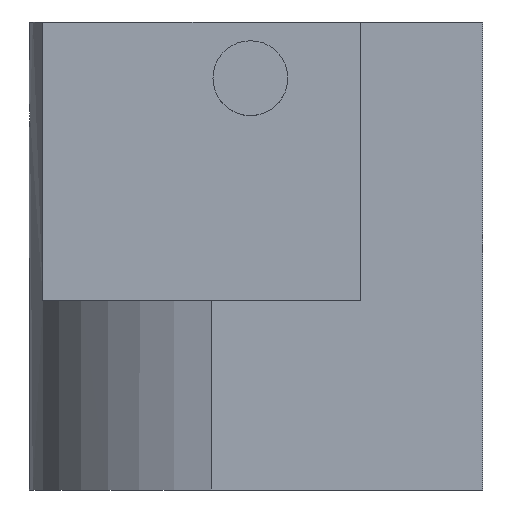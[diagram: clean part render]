
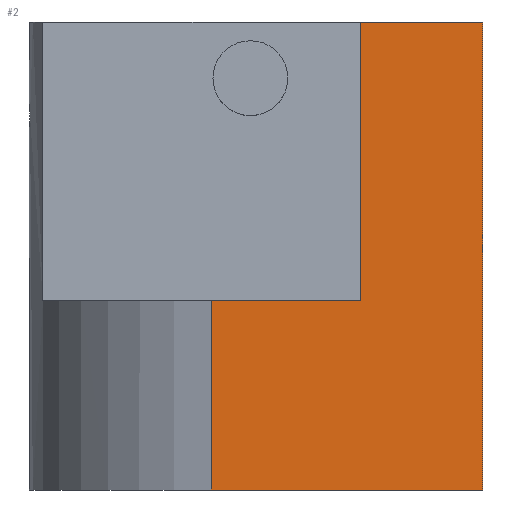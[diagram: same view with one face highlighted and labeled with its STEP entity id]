
A CAD part, left-side view. The second image highlights one B-rep face of the part: STEP entity #2.
In plain terms, the highlighted planar face has unit normal (-1, 0, 0).
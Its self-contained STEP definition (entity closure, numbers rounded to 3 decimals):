
#2 = ADVANCED_FACE ( 'NONE', ( #112 ), #1020, .F. ) ;
#26 = ORIENTED_EDGE ( 'NONE', *, *, #1511, .F. ) ;
#98 = VERTEX_POINT ( 'NONE', #1521 ) ;
#99 = LINE ( 'NONE', #606, #130 ) ;
#102 = DIRECTION ( 'NONE',  ( 0., 0., 1. ) ) ;
#106 = EDGE_LOOP ( 'NONE', ( #1433, #1058, #26, #1536, #1335, #1296 ) ) ;
#112 = FACE_OUTER_BOUND ( 'NONE', #106, .T. ) ;
#130 = VECTOR ( 'NONE', #1108, 1000. ) ;
#151 = CARTESIAN_POINT ( 'NONE',  ( -58.909, 11.39, -190. ) ) ;
#162 = CARTESIAN_POINT ( 'NONE',  ( -58.909, 11.39, -190. ) ) ;
#211 = DIRECTION ( 'NONE',  ( 0., 1., 0. ) ) ;
#288 = CARTESIAN_POINT ( 'NONE',  ( -58.909, -61., -65. ) ) ;
#294 = LINE ( 'NONE', #162, #819 ) ;
#301 = LINE ( 'NONE', #151, #1071 ) ;
#314 = VECTOR ( 'NONE', #211, 1000. ) ;
#342 = VERTEX_POINT ( 'NONE', #598 ) ;
#349 = CARTESIAN_POINT ( 'NONE',  ( -58.909, -28.313, -40. ) ) ;
#363 = AXIS2_PLACEMENT_3D ( 'NONE', #1121, #1144, #387 ) ;
#370 = EDGE_CURVE ( 'NONE', #1182, #448, #1351, .T. ) ;
#387 = DIRECTION ( 'NONE',  ( 0., 1., 0. ) ) ;
#395 = DIRECTION ( 'NONE',  ( 0., -1., 0. ) ) ;
#397 = VERTEX_POINT ( 'NONE', #1469 ) ;
#448 = VERTEX_POINT ( 'NONE', #887 ) ;
#529 = EDGE_CURVE ( 'NONE', #342, #1325, #294, .T. ) ;
#552 = DIRECTION ( 'NONE',  ( 0., 1., 0. ) ) ;
#598 = CARTESIAN_POINT ( 'NONE',  ( -58.909, -61., -190. ) ) ;
#606 = CARTESIAN_POINT ( 'NONE',  ( -58.909, -61., -190. ) ) ;
#780 = EDGE_CURVE ( 'NONE', #342, #1182, #99, .T. ) ;
#819 = VECTOR ( 'NONE', #552, 1000. ) ;
#821 = VECTOR ( 'NONE', #395, 1000. ) ;
#834 = CARTESIAN_POINT ( 'NONE',  ( -58.909, 11.39, -65. ) ) ;
#887 = CARTESIAN_POINT ( 'NONE',  ( -58.909, -28.313, -65. ) ) ;
#1019 = CARTESIAN_POINT ( 'NONE',  ( -58.909, -28.313, -139.424 ) ) ;
#1020 = PLANE ( 'NONE',  #363 ) ;
#1058 = ORIENTED_EDGE ( 'NONE', *, *, #1318, .F. ) ;
#1071 = VECTOR ( 'NONE', #1309, 1000. ) ;
#1108 = DIRECTION ( 'NONE',  ( 0., 0., 1. ) ) ;
#1121 = CARTESIAN_POINT ( 'NONE',  ( -58.909, 11.39, -190. ) ) ;
#1135 = LINE ( 'NONE', #1019, #821 ) ;
#1144 = DIRECTION ( 'NONE',  ( 1., 0., 0. ) ) ;
#1182 = VERTEX_POINT ( 'NONE', #288 ) ;
#1199 = CARTESIAN_POINT ( 'NONE',  ( -58.909, 11.39, -190. ) ) ;
#1296 = ORIENTED_EDGE ( 'NONE', *, *, #780, .T. ) ;
#1309 = DIRECTION ( 'NONE',  ( 0., 0., 1. ) ) ;
#1318 = EDGE_CURVE ( 'NONE', #397, #448, #1455, .T. ) ;
#1325 = VERTEX_POINT ( 'NONE', #1199 ) ;
#1335 = ORIENTED_EDGE ( 'NONE', *, *, #529, .F. ) ;
#1351 = LINE ( 'NONE', #834, #314 ) ;
#1433 = ORIENTED_EDGE ( 'NONE', *, *, #370, .T. ) ;
#1455 = LINE ( 'NONE', #349, #1461 ) ;
#1461 = VECTOR ( 'NONE', #102, 1000. ) ;
#1469 = CARTESIAN_POINT ( 'NONE',  ( -58.909, -28.313, -139.424 ) ) ;
#1511 = EDGE_CURVE ( 'NONE', #98, #397, #1135, .T. ) ;
#1521 = CARTESIAN_POINT ( 'NONE',  ( -58.909, 11.39, -139.424 ) ) ;
#1536 = ORIENTED_EDGE ( 'NONE', *, *, #1612, .F. ) ;
#1612 = EDGE_CURVE ( 'NONE', #1325, #98, #301, .T. ) ;
